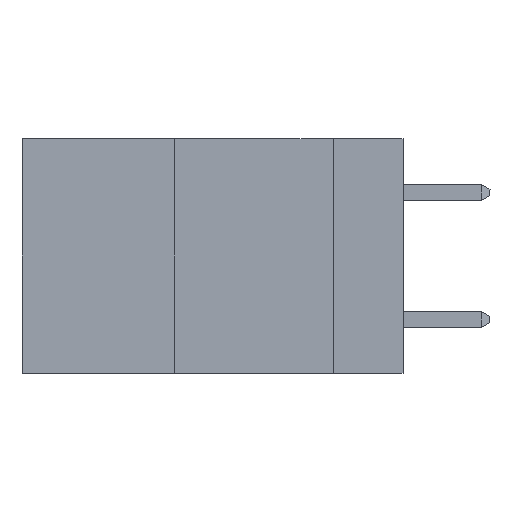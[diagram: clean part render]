
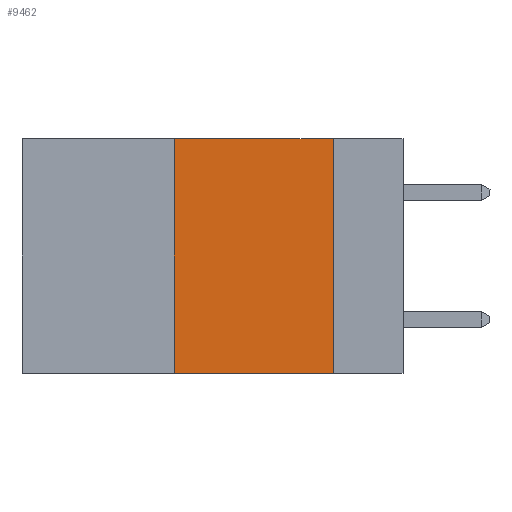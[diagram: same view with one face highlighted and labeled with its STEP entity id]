
A CAD part, left-side view. The second image highlights one B-rep face of the part: STEP entity #9462.
In plain terms, the highlighted planar face has unit normal (-1, 0, 0).
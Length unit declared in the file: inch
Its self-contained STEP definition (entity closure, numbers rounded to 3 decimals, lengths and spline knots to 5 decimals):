
#56 = VERTEX_POINT ( 'NONE', #7783 ) ;
#747 = CARTESIAN_POINT ( 'NONE',  ( 0., 0.11, 0. ) ) ;
#1009 = LINE ( 'NONE', #1510, #11858 ) ;
#1121 = EDGE_CURVE ( 'NONE', #3929, #13397, #3013, .T. ) ;
#1510 = CARTESIAN_POINT ( 'NONE',  ( 0., 0.6, -0.37 ) ) ;
#1703 = ORIENTED_EDGE ( 'NONE', *, *, #10664, .T. ) ;
#2277 = EDGE_LOOP ( 'NONE', ( #12297, #11359, #13350, #1703 ) ) ;
#2517 = VECTOR ( 'NONE', #4173, 39.37008 ) ;
#2544 = CARTESIAN_POINT ( 'NONE',  ( 0., 0.11, -0.37 ) ) ;
#2611 = DIRECTION ( 'NONE',  ( 0., -1., 0. ) ) ;
#2863 = LINE ( 'NONE', #11471, #2517 ) ;
#3013 = LINE ( 'NONE', #747, #11341 ) ;
#3929 = VERTEX_POINT ( 'NONE', #5807 ) ;
#4158 = CARTESIAN_POINT ( 'NONE',  ( 0., 0.6, 0. ) ) ;
#4173 = DIRECTION ( 'NONE',  ( 0., -1., 0. ) ) ;
#5270 = DIRECTION ( 'NONE',  ( 0., 0., -1. ) ) ;
#5807 = CARTESIAN_POINT ( 'NONE',  ( 0., 0.11, 0. ) ) ;
#6618 = AXIS2_PLACEMENT_3D ( 'NONE', #4158, #11461, #5270 ) ;
#6686 = DIRECTION ( 'NONE',  ( 0., 0., -1. ) ) ;
#7403 = CARTESIAN_POINT ( 'NONE',  ( 0., 0.36, -0.37 ) ) ;
#7783 = CARTESIAN_POINT ( 'NONE',  ( 0., 0.36, 0. ) ) ;
#8057 = LINE ( 'NONE', #9955, #10818 ) ;
#8509 = EDGE_CURVE ( 'NONE', #9530, #56, #8057, .T. ) ;
#9462 = ADVANCED_FACE ( 'NONE', ( #11118 ), #13365, .F. ) ;
#9530 = VERTEX_POINT ( 'NONE', #7403 ) ;
#9955 = CARTESIAN_POINT ( 'NONE',  ( 0., 0.36, 0. ) ) ;
#10664 = EDGE_CURVE ( 'NONE', #9530, #13397, #1009, .T. ) ;
#10818 = VECTOR ( 'NONE', #10995, 39.37008 ) ;
#10995 = DIRECTION ( 'NONE',  ( 0., 0., 1. ) ) ;
#11118 = FACE_OUTER_BOUND ( 'NONE', #2277, .T. ) ;
#11341 = VECTOR ( 'NONE', #6686, 39.37008 ) ;
#11359 = ORIENTED_EDGE ( 'NONE', *, *, #13065, .F. ) ;
#11461 = DIRECTION ( 'NONE',  ( 1., 0., 0. ) ) ;
#11471 = CARTESIAN_POINT ( 'NONE',  ( 0., 0.6, 0. ) ) ;
#11858 = VECTOR ( 'NONE', #2611, 39.37008 ) ;
#12297 = ORIENTED_EDGE ( 'NONE', *, *, #1121, .F. ) ;
#13065 = EDGE_CURVE ( 'NONE', #56, #3929, #2863, .T. ) ;
#13350 = ORIENTED_EDGE ( 'NONE', *, *, #8509, .F. ) ;
#13365 = PLANE ( 'NONE',  #6618 ) ;
#13397 = VERTEX_POINT ( 'NONE', #2544 ) ;
